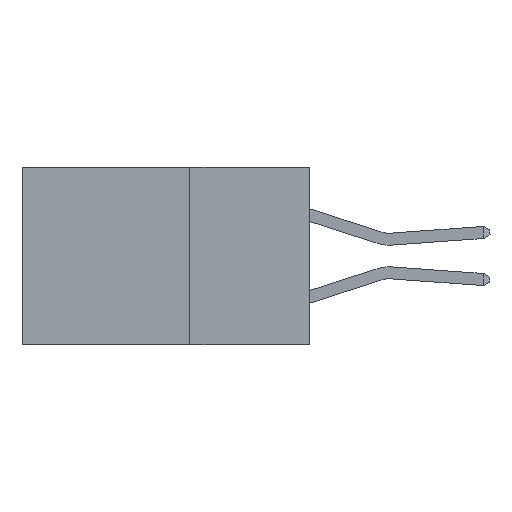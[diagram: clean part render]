
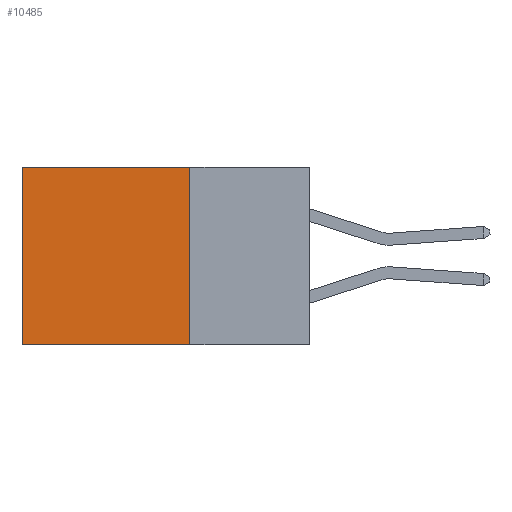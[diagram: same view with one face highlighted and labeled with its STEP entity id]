
A CAD part, left-side view. The second image highlights one B-rep face of the part: STEP entity #10485.
In plain terms, the highlighted planar face has unit normal (-1, 0, 0).
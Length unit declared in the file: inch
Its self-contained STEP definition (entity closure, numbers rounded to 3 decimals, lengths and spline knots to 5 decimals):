
#384 = EDGE_CURVE ( 'NONE', #5493, #2492, #13775, .T. ) ;
#1319 = PLANE ( 'NONE',  #7740 ) ;
#1568 = DIRECTION ( 'NONE',  ( 0., 0., -1. ) ) ;
#1717 = CARTESIAN_POINT ( 'NONE',  ( 0.298, 0.6, 0. ) ) ;
#1793 = VECTOR ( 'NONE', #1568, 39.37008 ) ;
#2492 = VERTEX_POINT ( 'NONE', #4202 ) ;
#2535 = EDGE_CURVE ( 'NONE', #15734, #5493, #3930, .T. ) ;
#2599 = CARTESIAN_POINT ( 'NONE',  ( 0.298, 0.25, 0. ) ) ;
#3287 = CARTESIAN_POINT ( 'NONE',  ( 0.298, 0.25, 0. ) ) ;
#3462 = EDGE_CURVE ( 'NONE', #15734, #10166, #12475, .T. ) ;
#3540 = VECTOR ( 'NONE', #8113, 39.37008 ) ;
#3613 = VECTOR ( 'NONE', #3770, 39.37008 ) ;
#3770 = DIRECTION ( 'NONE',  ( 0., 1., 0. ) ) ;
#3849 = DIRECTION ( 'NONE',  ( 0., 0., -1. ) ) ;
#3930 = LINE ( 'NONE', #11661, #3540 ) ;
#4202 = CARTESIAN_POINT ( 'NONE',  ( 0.298, 0.6, -0.37 ) ) ;
#4502 = EDGE_LOOP ( 'NONE', ( #12463, #5662, #12054, #8744 ) ) ;
#5493 = VERTEX_POINT ( 'NONE', #7243 ) ;
#5662 = ORIENTED_EDGE ( 'NONE', *, *, #384, .F. ) ;
#7243 = CARTESIAN_POINT ( 'NONE',  ( 0.298, 0.25, -0.37 ) ) ;
#7581 = CARTESIAN_POINT ( 'NONE',  ( 0.298, 0.25, -0.37 ) ) ;
#7740 = AXIS2_PLACEMENT_3D ( 'NONE', #2599, #11471, #3849 ) ;
#7914 = EDGE_CURVE ( 'NONE', #10166, #2492, #11508, .T. ) ;
#8113 = DIRECTION ( 'NONE',  ( 0., 0., -1. ) ) ;
#8364 = DIRECTION ( 'NONE',  ( 0., 1., 0. ) ) ;
#8744 = ORIENTED_EDGE ( 'NONE', *, *, #3462, .T. ) ;
#9172 = CARTESIAN_POINT ( 'NONE',  ( 0.298, 0.6, 0. ) ) ;
#10166 = VERTEX_POINT ( 'NONE', #1717 ) ;
#10485 = ADVANCED_FACE ( 'NONE', ( #10835 ), #1319, .F. ) ;
#10835 = FACE_OUTER_BOUND ( 'NONE', #4502, .T. ) ;
#10945 = CARTESIAN_POINT ( 'NONE',  ( 0.298, 0.25, 0. ) ) ;
#11471 = DIRECTION ( 'NONE',  ( 1., 0., 0. ) ) ;
#11508 = LINE ( 'NONE', #9172, #1793 ) ;
#11661 = CARTESIAN_POINT ( 'NONE',  ( 0.298, 0.25, 0. ) ) ;
#12054 = ORIENTED_EDGE ( 'NONE', *, *, #2535, .F. ) ;
#12082 = VECTOR ( 'NONE', #8364, 39.37008 ) ;
#12463 = ORIENTED_EDGE ( 'NONE', *, *, #7914, .T. ) ;
#12475 = LINE ( 'NONE', #3287, #12082 ) ;
#13775 = LINE ( 'NONE', #7581, #3613 ) ;
#15734 = VERTEX_POINT ( 'NONE', #10945 ) ;
